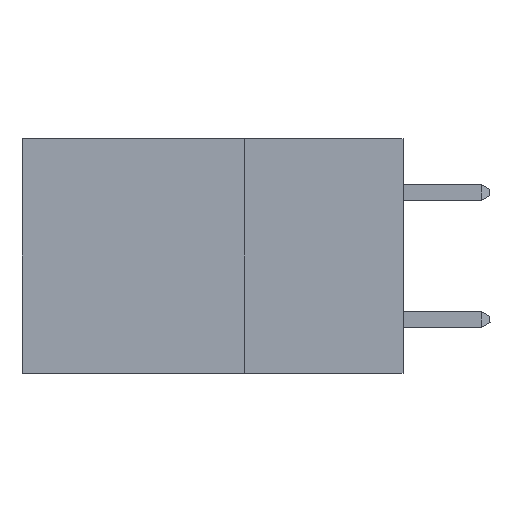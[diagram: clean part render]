
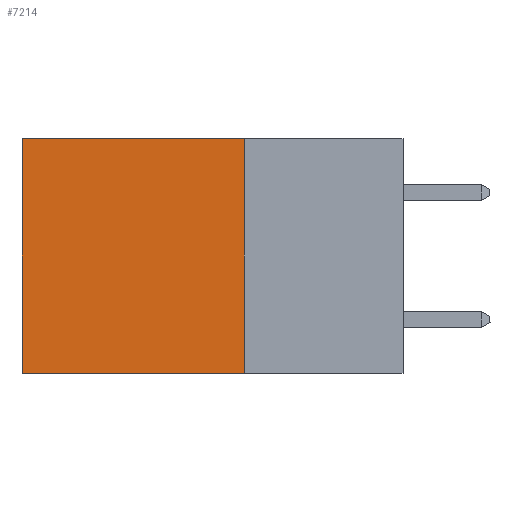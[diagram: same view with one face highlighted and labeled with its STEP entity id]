
A CAD part, left-side view. The second image highlights one B-rep face of the part: STEP entity #7214.
In plain terms, the highlighted planar face has unit normal (-1, 0, 0).
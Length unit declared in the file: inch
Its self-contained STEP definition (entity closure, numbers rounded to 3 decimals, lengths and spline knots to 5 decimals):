
#193 = PLANE ( 'NONE',  #27830 ) ;
#225 = DIRECTION ( 'NONE',  ( 0., 0., -1. ) ) ;
#3753 = VERTEX_POINT ( 'NONE', #28473 ) ;
#4031 = VECTOR ( 'NONE', #5952, 39.37008 ) ;
#5285 = EDGE_CURVE ( 'NONE', #8293, #3753, #26774, .T. ) ;
#5952 = DIRECTION ( 'NONE',  ( 0., 1., 0. ) ) ;
#6067 = CARTESIAN_POINT ( 'NONE',  ( 0.2875, 0.25, -0.37 ) ) ;
#7214 = ADVANCED_FACE ( 'NONE', ( #14016 ), #193, .F. ) ;
#7527 = VECTOR ( 'NONE', #23736, 39.37008 ) ;
#8205 = CARTESIAN_POINT ( 'NONE',  ( 0.2875, 0.25, 0. ) ) ;
#8293 = VERTEX_POINT ( 'NONE', #12452 ) ;
#9443 = VECTOR ( 'NONE', #18935, 39.37008 ) ;
#10366 = CARTESIAN_POINT ( 'NONE',  ( 0.2875, 0.6, 0. ) ) ;
#10855 = ORIENTED_EDGE ( 'NONE', *, *, #16188, .T. ) ;
#10945 = CARTESIAN_POINT ( 'NONE',  ( 0.2875, 0.25, 0. ) ) ;
#11515 = ORIENTED_EDGE ( 'NONE', *, *, #26350, .F. ) ;
#11528 = ORIENTED_EDGE ( 'NONE', *, *, #29090, .T. ) ;
#11975 = CARTESIAN_POINT ( 'NONE',  ( 0.2875, 0.6, -0.37 ) ) ;
#12452 = CARTESIAN_POINT ( 'NONE',  ( 0.2875, 0.25, 0. ) ) ;
#12518 = VERTEX_POINT ( 'NONE', #12539 ) ;
#12539 = CARTESIAN_POINT ( 'NONE',  ( 0.2875, 0.6, 0. ) ) ;
#13134 = CARTESIAN_POINT ( 'NONE',  ( 0.2875, 0.25, 0. ) ) ;
#13342 = VECTOR ( 'NONE', #35295, 39.37008 ) ;
#14016 = FACE_OUTER_BOUND ( 'NONE', #30362, .T. ) ;
#14189 = DIRECTION ( 'NONE',  ( 1., 0., 0. ) ) ;
#14236 = LINE ( 'NONE', #13134, #13342 ) ;
#14263 = LINE ( 'NONE', #10366, #9443 ) ;
#15382 = LINE ( 'NONE', #6067, #4031 ) ;
#16188 = EDGE_CURVE ( 'NONE', #12518, #25797, #14263, .T. ) ;
#18935 = DIRECTION ( 'NONE',  ( 0., 0., -1. ) ) ;
#23736 = DIRECTION ( 'NONE',  ( 0., 0., -1. ) ) ;
#25797 = VERTEX_POINT ( 'NONE', #11975 ) ;
#26350 = EDGE_CURVE ( 'NONE', #3753, #25797, #15382, .T. ) ;
#26774 = LINE ( 'NONE', #10945, #7527 ) ;
#27830 = AXIS2_PLACEMENT_3D ( 'NONE', #8205, #14189, #225 ) ;
#28473 = CARTESIAN_POINT ( 'NONE',  ( 0.2875, 0.25, -0.37 ) ) ;
#29090 = EDGE_CURVE ( 'NONE', #8293, #12518, #14236, .T. ) ;
#30362 = EDGE_LOOP ( 'NONE', ( #10855, #11515, #33715, #11528 ) ) ;
#33715 = ORIENTED_EDGE ( 'NONE', *, *, #5285, .F. ) ;
#35295 = DIRECTION ( 'NONE',  ( 0., 1., 0. ) ) ;
